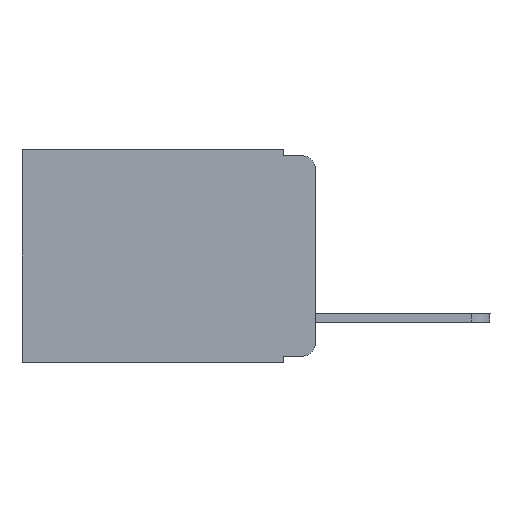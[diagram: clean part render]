
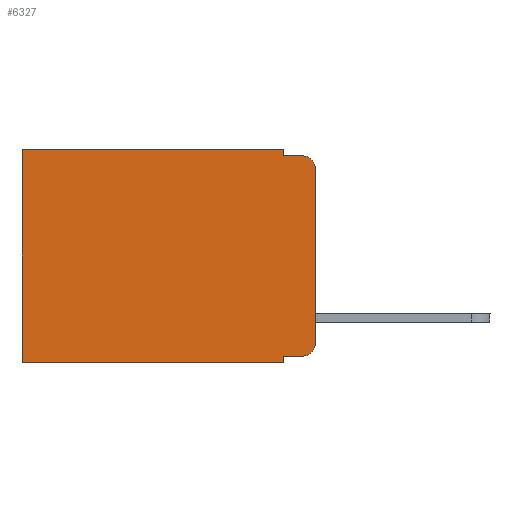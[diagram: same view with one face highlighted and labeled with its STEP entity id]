
A CAD part, left-side view. The second image highlights one B-rep face of the part: STEP entity #6327.
In plain terms, the highlighted planar face has unit normal (-1, 0, 0).
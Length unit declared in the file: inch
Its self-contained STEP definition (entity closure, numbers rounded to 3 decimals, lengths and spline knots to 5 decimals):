
#1261 = LINE ( 'NONE', #24243, #23048 ) ;
#1564 = VECTOR ( 'NONE', #17836, 39.37008 ) ;
#1925 = FACE_OUTER_BOUND ( 'NONE', #20909, .T. ) ;
#1962 = DIRECTION ( 'NONE',  ( 0., 1., 0. ) ) ;
#2079 = LINE ( 'NONE', #3839, #5174 ) ;
#2573 = VERTEX_POINT ( 'NONE', #6973 ) ;
#2656 = VERTEX_POINT ( 'NONE', #12686 ) ;
#2726 = CARTESIAN_POINT ( 'NONE',  ( 0.298, 0.051, 0. ) ) ;
#3690 = LINE ( 'NONE', #20787, #17921 ) ;
#3839 = CARTESIAN_POINT ( 'NONE',  ( 0.298, 0., -0.343 ) ) ;
#3944 = ORIENTED_EDGE ( 'NONE', *, *, #15707, .T. ) ;
#3999 = DIRECTION ( 'NONE',  ( -1., 0., 0. ) ) ;
#4306 = DIRECTION ( 'NONE',  ( 0., 0., -1. ) ) ;
#4389 = DIRECTION ( 'NONE',  ( -1., 0., 0. ) ) ;
#4466 = CARTESIAN_POINT ( 'NONE',  ( 0.298, 0.051, 0. ) ) ;
#4659 = EDGE_CURVE ( 'NONE', #23450, #2573, #9327, .T. ) ;
#5174 = VECTOR ( 'NONE', #1962, 39.37008 ) ;
#5236 = EDGE_CURVE ( 'NONE', #21622, #14352, #5243, .T. ) ;
#5243 = CIRCLE ( 'NONE', #7245, 0.02 ) ;
#5855 = CARTESIAN_POINT ( 'NONE',  ( 0.298, 0.02, -0.03 ) ) ;
#6327 = ADVANCED_FACE ( 'NONE', ( #1925 ), #17058, .F. ) ;
#6694 = LINE ( 'NONE', #14446, #17764 ) ;
#6717 = CARTESIAN_POINT ( 'NONE',  ( 0.298, 0., 0. ) ) ;
#6766 = EDGE_CURVE ( 'NONE', #22970, #20765, #10894, .T. ) ;
#6818 = CARTESIAN_POINT ( 'NONE',  ( 0.298, 0.473, -0.343 ) ) ;
#6973 = CARTESIAN_POINT ( 'NONE',  ( 0.298, 0.051, -0.343 ) ) ;
#7230 = ORIENTED_EDGE ( 'NONE', *, *, #4659, .F. ) ;
#7245 = AXIS2_PLACEMENT_3D ( 'NONE', #21735, #4389, #8253 ) ;
#7542 = DIRECTION ( 'NONE',  ( 1., 0., 0. ) ) ;
#7695 = AXIS2_PLACEMENT_3D ( 'NONE', #5855, #3999, #18872 ) ;
#8034 = CARTESIAN_POINT ( 'NONE',  ( 0.298, 0.051, 0. ) ) ;
#8061 = EDGE_CURVE ( 'NONE', #23765, #10402, #10459, .T. ) ;
#8253 = DIRECTION ( 'NONE',  ( 0., 0., -1. ) ) ;
#8486 = LINE ( 'NONE', #6717, #22051 ) ;
#9327 = LINE ( 'NONE', #8034, #18788 ) ;
#10402 = VERTEX_POINT ( 'NONE', #23990 ) ;
#10459 = LINE ( 'NONE', #4466, #1564 ) ;
#10894 = CIRCLE ( 'NONE', #7695, 0.02 ) ;
#11570 = VERTEX_POINT ( 'NONE', #6818 ) ;
#12686 = CARTESIAN_POINT ( 'NONE',  ( 0.298, 0.473, 0. ) ) ;
#12936 = CARTESIAN_POINT ( 'NONE',  ( 0.298, 0., -0.03 ) ) ;
#13598 = ORIENTED_EDGE ( 'NONE', *, *, #24075, .F. ) ;
#13686 = EDGE_CURVE ( 'NONE', #22970, #14352, #14162, .T. ) ;
#14045 = CARTESIAN_POINT ( 'NONE',  ( 0.298, 0., 0. ) ) ;
#14063 = CARTESIAN_POINT ( 'NONE',  ( 0.298, 0.02, -0.333 ) ) ;
#14162 = LINE ( 'NONE', #14045, #14588 ) ;
#14235 = DIRECTION ( 'NONE',  ( 0., 1., 0. ) ) ;
#14352 = VERTEX_POINT ( 'NONE', #15830 ) ;
#14446 = CARTESIAN_POINT ( 'NONE',  ( 0.298, 0.051, -0.01 ) ) ;
#14588 = VECTOR ( 'NONE', #4306, 39.37008 ) ;
#15540 = CARTESIAN_POINT ( 'NONE',  ( 0.298, 0.02, -0.01 ) ) ;
#15707 = EDGE_CURVE ( 'NONE', #23765, #2656, #8486, .T. ) ;
#15830 = CARTESIAN_POINT ( 'NONE',  ( 0.298, 0., -0.313 ) ) ;
#16482 = ORIENTED_EDGE ( 'NONE', *, *, #22909, .T. ) ;
#16839 = DIRECTION ( 'NONE',  ( 0., 0., -1. ) ) ;
#17058 = PLANE ( 'NONE',  #21170 ) ;
#17347 = ORIENTED_EDGE ( 'NONE', *, *, #5236, .T. ) ;
#17387 = EDGE_CURVE ( 'NONE', #10402, #20765, #6694, .T. ) ;
#17764 = VECTOR ( 'NONE', #20189, 39.37008 ) ;
#17836 = DIRECTION ( 'NONE',  ( 0., 0., -1. ) ) ;
#17921 = VECTOR ( 'NONE', #24419, 39.37008 ) ;
#18521 = DIRECTION ( 'NONE',  ( 0., 0., -1. ) ) ;
#18549 = DIRECTION ( 'NONE',  ( 0., 0., -1. ) ) ;
#18730 = ORIENTED_EDGE ( 'NONE', *, *, #6766, .T. ) ;
#18788 = VECTOR ( 'NONE', #16839, 39.37008 ) ;
#18872 = DIRECTION ( 'NONE',  ( 0., 0., -1. ) ) ;
#19858 = ORIENTED_EDGE ( 'NONE', *, *, #8061, .F. ) ;
#20189 = DIRECTION ( 'NONE',  ( 0., -1., 0. ) ) ;
#20765 = VERTEX_POINT ( 'NONE', #15540 ) ;
#20787 = CARTESIAN_POINT ( 'NONE',  ( 0.298, 0.051, -0.333 ) ) ;
#20909 = EDGE_LOOP ( 'NONE', ( #23983, #18730, #22519, #19858, #3944, #21180, #13598, #7230, #16482, #17347 ) ) ;
#21170 = AXIS2_PLACEMENT_3D ( 'NONE', #24651, #7542, #18549 ) ;
#21180 = ORIENTED_EDGE ( 'NONE', *, *, #22170, .T. ) ;
#21622 = VERTEX_POINT ( 'NONE', #14063 ) ;
#21735 = CARTESIAN_POINT ( 'NONE',  ( 0.298, 0.02, -0.313 ) ) ;
#22051 = VECTOR ( 'NONE', #14235, 39.37008 ) ;
#22170 = EDGE_CURVE ( 'NONE', #2656, #11570, #1261, .T. ) ;
#22519 = ORIENTED_EDGE ( 'NONE', *, *, #17387, .F. ) ;
#22909 = EDGE_CURVE ( 'NONE', #23450, #21622, #3690, .T. ) ;
#22970 = VERTEX_POINT ( 'NONE', #12936 ) ;
#23048 = VECTOR ( 'NONE', #18521, 39.37008 ) ;
#23450 = VERTEX_POINT ( 'NONE', #24352 ) ;
#23765 = VERTEX_POINT ( 'NONE', #2726 ) ;
#23983 = ORIENTED_EDGE ( 'NONE', *, *, #13686, .F. ) ;
#23990 = CARTESIAN_POINT ( 'NONE',  ( 0.298, 0.051, -0.01 ) ) ;
#24075 = EDGE_CURVE ( 'NONE', #2573, #11570, #2079, .T. ) ;
#24243 = CARTESIAN_POINT ( 'NONE',  ( 0.298, 0.473, 0. ) ) ;
#24352 = CARTESIAN_POINT ( 'NONE',  ( 0.298, 0.051, -0.333 ) ) ;
#24419 = DIRECTION ( 'NONE',  ( 0., -1., 0. ) ) ;
#24651 = CARTESIAN_POINT ( 'NONE',  ( 0.298, 0., 0. ) ) ;
